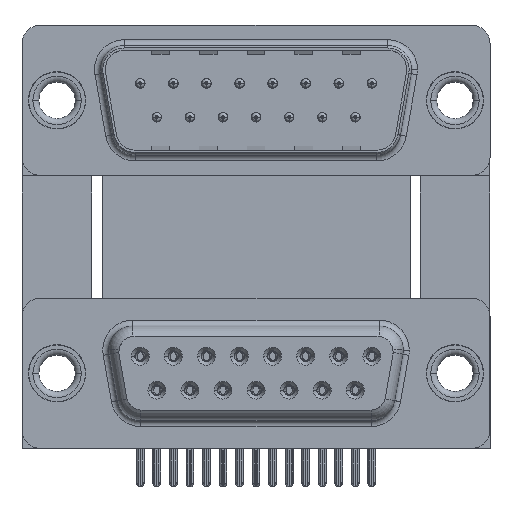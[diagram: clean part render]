
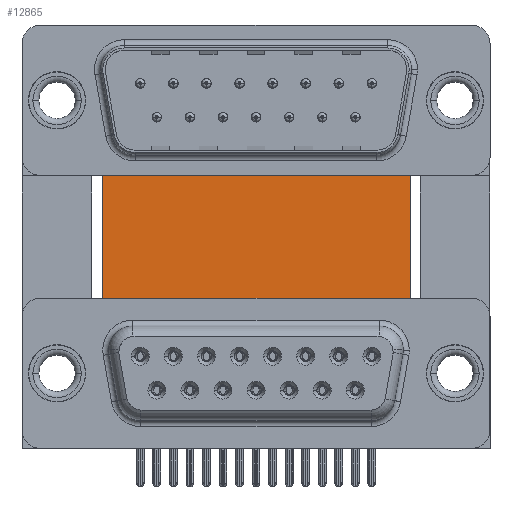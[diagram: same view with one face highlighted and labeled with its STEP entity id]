
A CAD part, top view. The second image highlights one B-rep face of the part: STEP entity #12865.
In plain terms, the highlighted planar face has unit normal (0, 0, 1).
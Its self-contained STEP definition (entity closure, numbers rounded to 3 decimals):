
#54 = ORIENTED_EDGE ( 'NONE', *, *, #8892, .F. ) ;
#1671 = VERTEX_POINT ( 'NONE', #9848 ) ;
#2671 = CARTESIAN_POINT ( 'NONE',  ( 3.79, 16.585, -12. ) ) ;
#2701 = VERTEX_POINT ( 'NONE', #22097 ) ;
#3556 = DIRECTION ( 'NONE',  ( 0., -1., 0. ) ) ;
#4939 = LINE ( 'NONE', #14709, #41395 ) ;
#5154 = VECTOR ( 'NONE', #33229, 1000. ) ;
#8892 = EDGE_CURVE ( 'NONE', #26761, #2701, #4939, .T. ) ;
#9553 = CARTESIAN_POINT ( 'NONE',  ( 3.79, -3.735, -12. ) ) ;
#9827 = AXIS2_PLACEMENT_3D ( 'NONE', #20222, #27359, #34488 ) ;
#9848 = CARTESIAN_POINT ( 'NONE',  ( 29.58, -3.735, -12. ) ) ;
#10232 = FACE_OUTER_BOUND ( 'NONE', #20073, .T. ) ;
#10808 = CARTESIAN_POINT ( 'NONE',  ( 3.79, 16.585, -12. ) ) ;
#11565 = CARTESIAN_POINT ( 'NONE',  ( 3.79, -3.735, -12. ) ) ;
#12865 = ADVANCED_FACE ( 'NONE', ( #10232 ), #17097, .F. ) ;
#12973 = LINE ( 'NONE', #43933, #5154 ) ;
#14709 = CARTESIAN_POINT ( 'NONE',  ( 3.79, 16.585, -12. ) ) ;
#16334 = VECTOR ( 'NONE', #21567, 1000. ) ;
#17097 = PLANE ( 'NONE',  #9827 ) ;
#17311 = ORIENTED_EDGE ( 'NONE', *, *, #32085, .T. ) ;
#17633 = EDGE_CURVE ( 'NONE', #26761, #40298, #40522, .T. ) ;
#17860 = ORIENTED_EDGE ( 'NONE', *, *, #17633, .T. ) ;
#20073 = EDGE_LOOP ( 'NONE', ( #17311, #43890, #54, #17860 ) ) ;
#20222 = CARTESIAN_POINT ( 'NONE',  ( 3.79, 16.585, -12. ) ) ;
#21479 = EDGE_CURVE ( 'NONE', #2701, #1671, #12973, .T. ) ;
#21567 = DIRECTION ( 'NONE',  ( 1., 0., 0. ) ) ;
#22097 = CARTESIAN_POINT ( 'NONE',  ( 29.58, 16.585, -12. ) ) ;
#26761 = VERTEX_POINT ( 'NONE', #2671 ) ;
#27359 = DIRECTION ( 'NONE',  ( 0., 0., -1. ) ) ;
#32085 = EDGE_CURVE ( 'NONE', #40298, #1671, #38522, .T. ) ;
#33229 = DIRECTION ( 'NONE',  ( 0., -1., 0. ) ) ;
#34488 = DIRECTION ( 'NONE',  ( -1., 0., 0. ) ) ;
#38522 = LINE ( 'NONE', #11565, #16334 ) ;
#38765 = DIRECTION ( 'NONE',  ( 1., 0., 0. ) ) ;
#40298 = VERTEX_POINT ( 'NONE', #9553 ) ;
#40522 = LINE ( 'NONE', #10808, #43407 ) ;
#41395 = VECTOR ( 'NONE', #38765, 1000. ) ;
#43407 = VECTOR ( 'NONE', #3556, 1000. ) ;
#43890 = ORIENTED_EDGE ( 'NONE', *, *, #21479, .F. ) ;
#43933 = CARTESIAN_POINT ( 'NONE',  ( 29.58, 16.585, -12. ) ) ;
